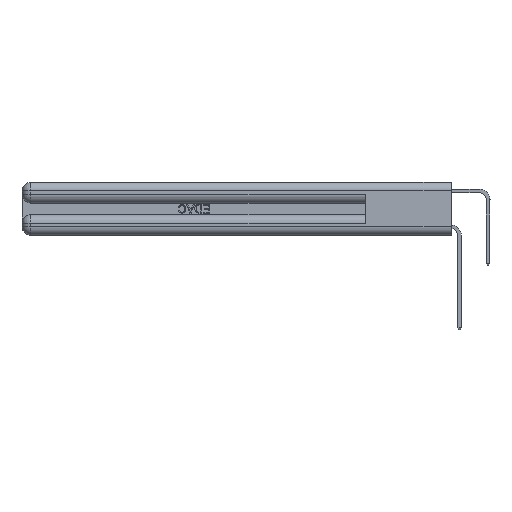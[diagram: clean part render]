
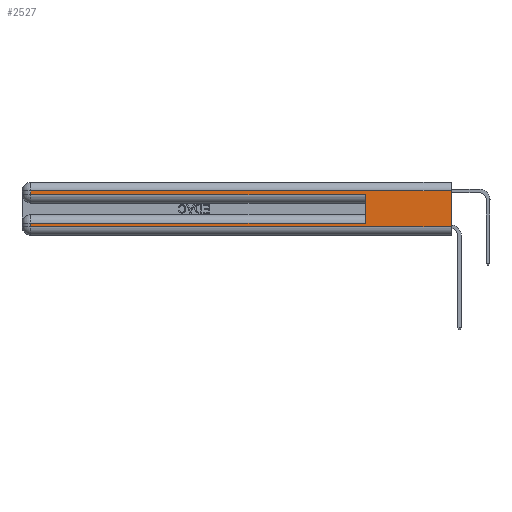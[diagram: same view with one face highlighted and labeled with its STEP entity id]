
A CAD part, left-side view. The second image highlights one B-rep face of the part: STEP entity #2527.
In plain terms, the highlighted planar face has unit normal (-1, 0, 0).
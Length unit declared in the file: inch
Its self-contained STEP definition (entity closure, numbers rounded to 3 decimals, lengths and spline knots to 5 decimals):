
#154 = EDGE_CURVE ( 'NONE', #4041, #10698, #16027, .T. ) ;
#704 = CARTESIAN_POINT ( 'NONE',  ( 0., 2.94, 0.285 ) ) ;
#1101 = VERTEX_POINT ( 'NONE', #704 ) ;
#2453 = CARTESIAN_POINT ( 'NONE',  ( 0., 2.94, 0.31 ) ) ;
#2527 = ADVANCED_FACE ( 'NONE', ( #7915 ), #19414, .F. ) ;
#2935 = LINE ( 'NONE', #28071, #17688 ) ;
#3172 = DIRECTION ( 'NONE',  ( 1., 0., 0. ) ) ;
#3303 = EDGE_CURVE ( 'NONE', #34609, #10698, #34565, .T. ) ;
#3352 = CARTESIAN_POINT ( 'NONE',  ( 0., 2.94, 0.37 ) ) ;
#3688 = DIRECTION ( 'NONE',  ( 0., -1., 0. ) ) ;
#4041 = VERTEX_POINT ( 'NONE', #21075 ) ;
#4178 = VECTOR ( 'NONE', #6224, 39.37008 ) ;
#4967 = EDGE_CURVE ( 'NONE', #1101, #30559, #9545, .T. ) ;
#5924 = EDGE_LOOP ( 'NONE', ( #27941, #6286, #13723, #6536, #29094, #6504, #32440, #7507 ) ) ;
#6140 = CARTESIAN_POINT ( 'NONE',  ( 0., 0., 0.06 ) ) ;
#6224 = DIRECTION ( 'NONE',  ( 0., 1., 0. ) ) ;
#6286 = ORIENTED_EDGE ( 'NONE', *, *, #21406, .T. ) ;
#6504 = ORIENTED_EDGE ( 'NONE', *, *, #22893, .T. ) ;
#6536 = ORIENTED_EDGE ( 'NONE', *, *, #4967, .T. ) ;
#7507 = ORIENTED_EDGE ( 'NONE', *, *, #154, .T. ) ;
#7915 = FACE_OUTER_BOUND ( 'NONE', #5924, .T. ) ;
#8454 = VERTEX_POINT ( 'NONE', #31703 ) ;
#9060 = DIRECTION ( 'NONE',  ( 0., 0., -1. ) ) ;
#9266 = EDGE_CURVE ( 'NONE', #8454, #4041, #31192, .T. ) ;
#9545 = LINE ( 'NONE', #31598, #23049 ) ;
#10371 = DIRECTION ( 'NONE',  ( 0., -1., 0. ) ) ;
#10698 = VERTEX_POINT ( 'NONE', #13176 ) ;
#11334 = LINE ( 'NONE', #16967, #4178 ) ;
#12151 = VECTOR ( 'NONE', #29830, 39.37008 ) ;
#12742 = EDGE_CURVE ( 'NONE', #31024, #1101, #12744, .T. ) ;
#12744 = LINE ( 'NONE', #28271, #33478 ) ;
#13176 = CARTESIAN_POINT ( 'NONE',  ( 0., 0., 0.06 ) ) ;
#13723 = ORIENTED_EDGE ( 'NONE', *, *, #12742, .T. ) ;
#14163 = CARTESIAN_POINT ( 'NONE',  ( 0., 0., 0.37 ) ) ;
#14406 = CARTESIAN_POINT ( 'NONE',  ( 0., 0.6, 0.085 ) ) ;
#15112 = LINE ( 'NONE', #16364, #12151 ) ;
#16027 = LINE ( 'NONE', #6140, #28687 ) ;
#16364 = CARTESIAN_POINT ( 'NONE',  ( 0., 0.6, 0.145 ) ) ;
#16967 = CARTESIAN_POINT ( 'NONE',  ( 0., 0., 0.085 ) ) ;
#17280 = VECTOR ( 'NONE', #33203, 39.37008 ) ;
#17688 = VECTOR ( 'NONE', #30661, 39.37008 ) ;
#18902 = VECTOR ( 'NONE', #32731, 39.37008 ) ;
#18922 = VERTEX_POINT ( 'NONE', #14406 ) ;
#19414 = PLANE ( 'NONE',  #22561 ) ;
#21075 = CARTESIAN_POINT ( 'NONE',  ( 0., 2.94, 0.06 ) ) ;
#21406 = EDGE_CURVE ( 'NONE', #34609, #31024, #2935, .T. ) ;
#21499 = CARTESIAN_POINT ( 'NONE',  ( 0., 0.6, 0.285 ) ) ;
#22175 = DIRECTION ( 'NONE',  ( 0., 0., -1. ) ) ;
#22561 = AXIS2_PLACEMENT_3D ( 'NONE', #27579, #3172, #22175 ) ;
#22682 = EDGE_CURVE ( 'NONE', #18922, #30559, #15112, .T. ) ;
#22893 = EDGE_CURVE ( 'NONE', #18922, #8454, #11334, .T. ) ;
#23049 = VECTOR ( 'NONE', #10371, 39.37008 ) ;
#27579 = CARTESIAN_POINT ( 'NONE',  ( 0., 0., 0.37 ) ) ;
#27941 = ORIENTED_EDGE ( 'NONE', *, *, #3303, .F. ) ;
#28071 = CARTESIAN_POINT ( 'NONE',  ( 0., 0., 0.31 ) ) ;
#28271 = CARTESIAN_POINT ( 'NONE',  ( 0., 2.94, 0.37 ) ) ;
#28687 = VECTOR ( 'NONE', #3688, 39.37008 ) ;
#29094 = ORIENTED_EDGE ( 'NONE', *, *, #22682, .F. ) ;
#29830 = DIRECTION ( 'NONE',  ( 0., 0., 1. ) ) ;
#30559 = VERTEX_POINT ( 'NONE', #21499 ) ;
#30661 = DIRECTION ( 'NONE',  ( 0., 1., 0. ) ) ;
#31024 = VERTEX_POINT ( 'NONE', #2453 ) ;
#31040 = CARTESIAN_POINT ( 'NONE',  ( 0., 0., 0.31 ) ) ;
#31192 = LINE ( 'NONE', #3352, #17280 ) ;
#31598 = CARTESIAN_POINT ( 'NONE',  ( 0., 0., 0.285 ) ) ;
#31703 = CARTESIAN_POINT ( 'NONE',  ( 0., 2.94, 0.085 ) ) ;
#32440 = ORIENTED_EDGE ( 'NONE', *, *, #9266, .T. ) ;
#32731 = DIRECTION ( 'NONE',  ( 0., 0., -1. ) ) ;
#33203 = DIRECTION ( 'NONE',  ( 0., 0., -1. ) ) ;
#33478 = VECTOR ( 'NONE', #9060, 39.37008 ) ;
#34565 = LINE ( 'NONE', #14163, #18902 ) ;
#34609 = VERTEX_POINT ( 'NONE', #31040 ) ;
